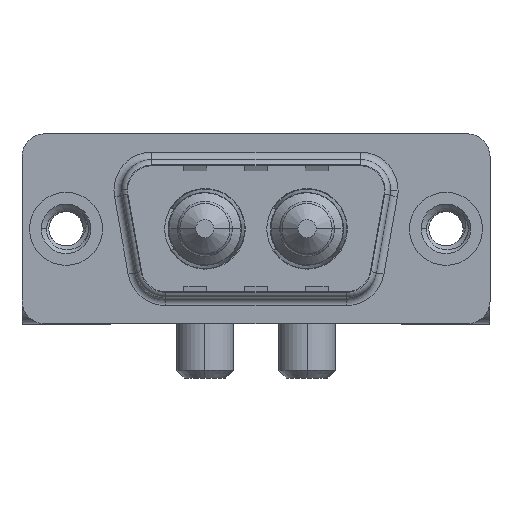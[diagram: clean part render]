
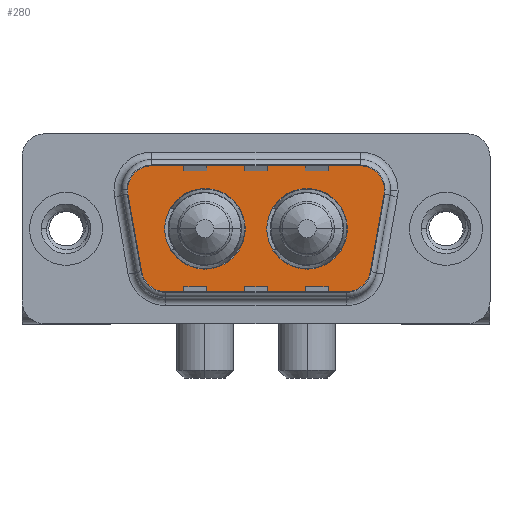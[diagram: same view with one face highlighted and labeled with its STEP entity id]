
A CAD part, top view. The second image highlights one B-rep face of the part: STEP entity #280.
In plain terms, the highlighted planar face has unit normal (0, 0, 1).
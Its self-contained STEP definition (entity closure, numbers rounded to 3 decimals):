
#12 = VERTEX_POINT ( 'NONE', #8639 ) ;
#84 = CARTESIAN_POINT ( 'NONE',  ( 9.14, 0., 0. ) ) ;
#140 = VERTEX_POINT ( 'NONE', #357 ) ;
#152 = DIRECTION ( 'NONE',  ( 1., 0., 0. ) ) ;
#199 = CIRCLE ( 'NONE', #9773, 2.65 ) ;
#246 = EDGE_CURVE ( 'NONE', #386, #12, #1817, .T. ) ;
#280 = ADVANCED_FACE ( 'NONE', ( #8389, #2790, #615 ), #2736, .T. ) ;
#333 = VERTEX_POINT ( 'NONE', #10146 ) ;
#357 = CARTESIAN_POINT ( 'NONE',  ( 6.459, -4.9, 0. ) ) ;
#386 = VERTEX_POINT ( 'NONE', #3025 ) ;
#395 = LINE ( 'NONE', #8065, #12133 ) ;
#513 = AXIS2_PLACEMENT_3D ( 'NONE', #11754, #7090, #9031 ) ;
#539 = DIRECTION ( 'NONE',  ( 0., 0., 1. ) ) ;
#576 = DIRECTION ( 'NONE',  ( 0., 0., 1. ) ) ;
#615 = FACE_OUTER_BOUND ( 'NONE', #6265, .T. ) ;
#628 = CARTESIAN_POINT ( 'NONE',  ( 6.459, -4.9, 0. ) ) ;
#682 = DIRECTION ( 'NONE',  ( 0.174, 0.985, 0. ) ) ;
#1143 = DIRECTION ( 'NONE',  ( 0., 0., 1. ) ) ;
#1157 = CARTESIAN_POINT ( 'NONE',  ( 11.79, 0., 0. ) ) ;
#1399 = DIRECTION ( 'NONE',  ( 0.174, -0.985, 0. ) ) ;
#1432 = EDGE_CURVE ( 'NONE', #5504, #11287, #6066, .T. ) ;
#1436 = EDGE_CURVE ( 'NONE', #140, #333, #4488, .T. ) ;
#1726 = CARTESIAN_POINT ( 'NONE',  ( 18.541, -2.9, 0. ) ) ;
#1817 = CIRCLE ( 'NONE', #10187, 2. ) ;
#1873 = CIRCLE ( 'NONE', #9640, 2. ) ;
#1912 = CIRCLE ( 'NONE', #10455, 2. ) ;
#2055 = EDGE_CURVE ( 'NONE', #333, #5504, #10421, .T. ) ;
#2345 = LINE ( 'NONE', #9070, #8520 ) ;
#2491 = AXIS2_PLACEMENT_3D ( 'NONE', #10643, #8527, #2855 ) ;
#2557 = DIRECTION ( 'NONE',  ( 1., 0., 0. ) ) ;
#2644 = CARTESIAN_POINT ( 'NONE',  ( 19.564, 2.9, 0. ) ) ;
#2699 = DIRECTION ( 'NONE',  ( 0., 0., 1. ) ) ;
#2736 = PLANE ( 'NONE',  #10777 ) ;
#2790 = FACE_BOUND ( 'NONE', #3986, .T. ) ;
#2855 = DIRECTION ( 'NONE',  ( 1., 0., 0. ) ) ;
#2858 = AXIS2_PLACEMENT_3D ( 'NONE', #10605, #1143, #9871 ) ;
#2940 = ORIENTED_EDGE ( 'NONE', *, *, #9432, .T. ) ;
#3025 = CARTESIAN_POINT ( 'NONE',  ( 21.564, 2.9, 0. ) ) ;
#3283 = AXIS2_PLACEMENT_3D ( 'NONE', #84, #8452, #152 ) ;
#3318 = CARTESIAN_POINT ( 'NONE',  ( 3.466, 2.553, 0. ) ) ;
#3339 = CARTESIAN_POINT ( 'NONE',  ( 6.459, -2.9, 0. ) ) ;
#3633 = CARTESIAN_POINT ( 'NONE',  ( 20.511, -3.247, 0. ) ) ;
#3863 = DIRECTION ( 'NONE',  ( 1., 0., 0. ) ) ;
#3981 = EDGE_CURVE ( 'NONE', #4516, #10048, #2345, .T. ) ;
#3986 = EDGE_LOOP ( 'NONE', ( #6484, #10417 ) ) ;
#4191 = CARTESIAN_POINT ( 'NONE',  ( 15.86, 0., 0. ) ) ;
#4302 = DIRECTION ( 'NONE',  ( 0., 0., 1. ) ) ;
#4471 = DIRECTION ( 'NONE',  ( 0., 0., 1. ) ) ;
#4481 = ORIENTED_EDGE ( 'NONE', *, *, #7091, .F. ) ;
#4488 = LINE ( 'NONE', #628, #8469 ) ;
#4516 = VERTEX_POINT ( 'NONE', #3318 ) ;
#4557 = CARTESIAN_POINT ( 'NONE',  ( 5.436, 2.9, 0. ) ) ;
#4577 = EDGE_LOOP ( 'NONE', ( #7256, #4481 ) ) ;
#4654 = CIRCLE ( 'NONE', #2491, 2.65 ) ;
#4690 = VECTOR ( 'NONE', #682, 1000. ) ;
#4952 = ORIENTED_EDGE ( 'NONE', *, *, #1432, .T. ) ;
#5152 = DIRECTION ( 'NONE',  ( -1., 0., 0. ) ) ;
#5504 = VERTEX_POINT ( 'NONE', #3633 ) ;
#5933 = CARTESIAN_POINT ( 'NONE',  ( 18.51, 0., 0. ) ) ;
#6066 = LINE ( 'NONE', #6306, #4690 ) ;
#6265 = EDGE_LOOP ( 'NONE', ( #8689, #4952, #6797, #6515, #12198, #6618, #6721, #2940, #10508 ) ) ;
#6293 = CARTESIAN_POINT ( 'NONE',  ( 19.564, 2.9, 0. ) ) ;
#6306 = CARTESIAN_POINT ( 'NONE',  ( 21.534, 2.553, 0. ) ) ;
#6484 = ORIENTED_EDGE ( 'NONE', *, *, #7900, .F. ) ;
#6502 = CARTESIAN_POINT ( 'NONE',  ( 4.489, -3.247, 0. ) ) ;
#6515 = ORIENTED_EDGE ( 'NONE', *, *, #246, .T. ) ;
#6606 = EDGE_CURVE ( 'NONE', #12, #9077, #395, .T. ) ;
#6618 = ORIENTED_EDGE ( 'NONE', *, *, #10567, .T. ) ;
#6721 = ORIENTED_EDGE ( 'NONE', *, *, #3981, .T. ) ;
#6797 = ORIENTED_EDGE ( 'NONE', *, *, #11814, .T. ) ;
#7090 = DIRECTION ( 'NONE',  ( 0., 0., 1. ) ) ;
#7091 = EDGE_CURVE ( 'NONE', #10796, #8373, #199, .T. ) ;
#7256 = ORIENTED_EDGE ( 'NONE', *, *, #11389, .F. ) ;
#7443 = EDGE_CURVE ( 'NONE', #7879, #11740, #4654, .T. ) ;
#7879 = VERTEX_POINT ( 'NONE', #11325 ) ;
#7900 = EDGE_CURVE ( 'NONE', #11740, #7879, #9242, .T. ) ;
#7938 = DIRECTION ( 'NONE',  ( -1., 0., 0. ) ) ;
#8065 = CARTESIAN_POINT ( 'NONE',  ( 5.436, 4.9, 0. ) ) ;
#8084 = AXIS2_PLACEMENT_3D ( 'NONE', #2644, #2699, #5152 ) ;
#8099 = DIRECTION ( 'NONE',  ( -1., 0., 0. ) ) ;
#8156 = CARTESIAN_POINT ( 'NONE',  ( 21.534, 2.553, 0. ) ) ;
#8354 = DIRECTION ( 'NONE',  ( 0., 0., 1. ) ) ;
#8373 = VERTEX_POINT ( 'NONE', #5933 ) ;
#8389 = FACE_BOUND ( 'NONE', #4577, .T. ) ;
#8452 = DIRECTION ( 'NONE',  ( 0., 0., 1. ) ) ;
#8469 = VECTOR ( 'NONE', #11105, 1000. ) ;
#8520 = VECTOR ( 'NONE', #1399, 1000. ) ;
#8527 = DIRECTION ( 'NONE',  ( 0., 0., 1. ) ) ;
#8639 = CARTESIAN_POINT ( 'NONE',  ( 19.564, 4.9, 0. ) ) ;
#8689 = ORIENTED_EDGE ( 'NONE', *, *, #2055, .T. ) ;
#9031 = DIRECTION ( 'NONE',  ( 1., 0., 0. ) ) ;
#9070 = CARTESIAN_POINT ( 'NONE',  ( 3.466, 2.553, 0. ) ) ;
#9077 = VERTEX_POINT ( 'NONE', #9974 ) ;
#9242 = CIRCLE ( 'NONE', #3283, 2.65 ) ;
#9432 = EDGE_CURVE ( 'NONE', #10048, #140, #1912, .T. ) ;
#9640 = AXIS2_PLACEMENT_3D ( 'NONE', #4557, #8354, #3863 ) ;
#9773 = AXIS2_PLACEMENT_3D ( 'NONE', #4191, #576, #11844 ) ;
#9871 = DIRECTION ( 'NONE',  ( 1., 0., 0. ) ) ;
#9974 = CARTESIAN_POINT ( 'NONE',  ( 5.436, 4.9, 0. ) ) ;
#10006 = DIRECTION ( 'NONE',  ( -1., 0., 0. ) ) ;
#10048 = VERTEX_POINT ( 'NONE', #6502 ) ;
#10146 = CARTESIAN_POINT ( 'NONE',  ( 18.541, -4.9, 0. ) ) ;
#10187 = AXIS2_PLACEMENT_3D ( 'NONE', #6293, #4302, #8099 ) ;
#10417 = ORIENTED_EDGE ( 'NONE', *, *, #7443, .F. ) ;
#10421 = CIRCLE ( 'NONE', #2858, 2. ) ;
#10455 = AXIS2_PLACEMENT_3D ( 'NONE', #3339, #539, #10006 ) ;
#10508 = ORIENTED_EDGE ( 'NONE', *, *, #1436, .T. ) ;
#10567 = EDGE_CURVE ( 'NONE', #9077, #4516, #1873, .T. ) ;
#10605 = CARTESIAN_POINT ( 'NONE',  ( 18.541, -2.9, 0. ) ) ;
#10643 = CARTESIAN_POINT ( 'NONE',  ( 9.14, 0., 0. ) ) ;
#10777 = AXIS2_PLACEMENT_3D ( 'NONE', #1726, #4471, #2557 ) ;
#10796 = VERTEX_POINT ( 'NONE', #11099 ) ;
#11099 = CARTESIAN_POINT ( 'NONE',  ( 13.21, 0., 0. ) ) ;
#11105 = DIRECTION ( 'NONE',  ( 1., 0., 0. ) ) ;
#11254 = CIRCLE ( 'NONE', #513, 2.65 ) ;
#11287 = VERTEX_POINT ( 'NONE', #8156 ) ;
#11325 = CARTESIAN_POINT ( 'NONE',  ( 6.49, 0., 0. ) ) ;
#11389 = EDGE_CURVE ( 'NONE', #8373, #10796, #11254, .T. ) ;
#11740 = VERTEX_POINT ( 'NONE', #1157 ) ;
#11754 = CARTESIAN_POINT ( 'NONE',  ( 15.86, 0., 0. ) ) ;
#11814 = EDGE_CURVE ( 'NONE', #11287, #386, #12045, .T. ) ;
#11844 = DIRECTION ( 'NONE',  ( 1., 0., 0. ) ) ;
#12045 = CIRCLE ( 'NONE', #8084, 2. ) ;
#12133 = VECTOR ( 'NONE', #7938, 1000. ) ;
#12198 = ORIENTED_EDGE ( 'NONE', *, *, #6606, .T. ) ;
